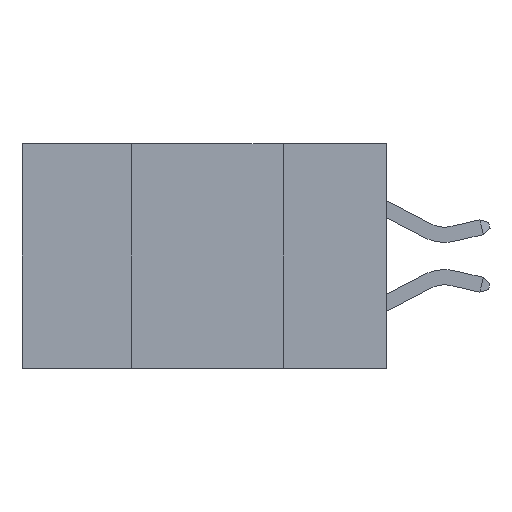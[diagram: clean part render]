
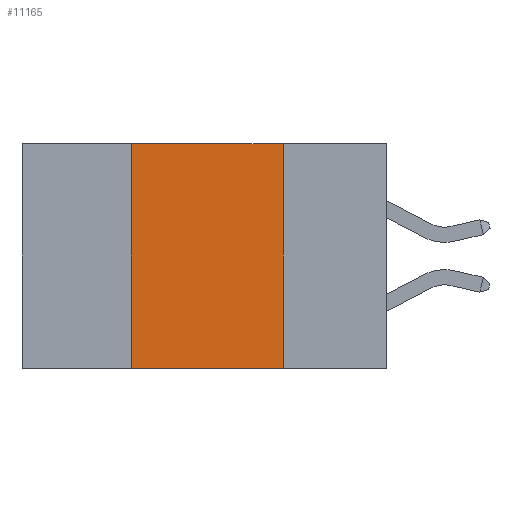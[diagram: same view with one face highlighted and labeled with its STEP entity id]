
A CAD part, left-side view. The second image highlights one B-rep face of the part: STEP entity #11165.
In plain terms, the highlighted planar face has unit normal (-1, 0, 0).
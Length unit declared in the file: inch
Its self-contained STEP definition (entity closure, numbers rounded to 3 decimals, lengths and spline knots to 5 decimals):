
#757 = VERTEX_POINT ( 'NONE', #3958 ) ;
#1578 = CARTESIAN_POINT ( 'NONE',  ( 0., 0.42, 0. ) ) ;
#1702 = LINE ( 'NONE', #13558, #7494 ) ;
#1704 = EDGE_LOOP ( 'NONE', ( #15202, #9391, #8829, #2153 ) ) ;
#2134 = CARTESIAN_POINT ( 'NONE',  ( 0., 0.6, 0. ) ) ;
#2153 = ORIENTED_EDGE ( 'NONE', *, *, #13921, .T. ) ;
#2189 = DIRECTION ( 'NONE',  ( 0., 0., -1. ) ) ;
#2686 = LINE ( 'NONE', #14157, #6401 ) ;
#3408 = DIRECTION ( 'NONE',  ( 1., 0., 0. ) ) ;
#3524 = VECTOR ( 'NONE', #10139, 39.37008 ) ;
#3958 = CARTESIAN_POINT ( 'NONE',  ( 0., 0.17, -0.37 ) ) ;
#5371 = CARTESIAN_POINT ( 'NONE',  ( 0., 0.6, -0.37 ) ) ;
#6296 = AXIS2_PLACEMENT_3D ( 'NONE', #2134, #3408, #11788 ) ;
#6401 = VECTOR ( 'NONE', #7159, 39.37008 ) ;
#6788 = LINE ( 'NONE', #5371, #3524 ) ;
#7139 = EDGE_CURVE ( 'NONE', #10209, #757, #11795, .T. ) ;
#7159 = DIRECTION ( 'NONE',  ( 0., 0., 1. ) ) ;
#7176 = VERTEX_POINT ( 'NONE', #11000 ) ;
#7494 = VECTOR ( 'NONE', #13507, 39.37008 ) ;
#7526 = CARTESIAN_POINT ( 'NONE',  ( 0., 0.17, 0. ) ) ;
#8829 = ORIENTED_EDGE ( 'NONE', *, *, #14829, .F. ) ;
#8831 = EDGE_CURVE ( 'NONE', #9405, #10209, #1702, .T. ) ;
#8929 = CARTESIAN_POINT ( 'NONE',  ( 0., 0.17, 0. ) ) ;
#9391 = ORIENTED_EDGE ( 'NONE', *, *, #8831, .F. ) ;
#9405 = VERTEX_POINT ( 'NONE', #1578 ) ;
#9433 = PLANE ( 'NONE',  #6296 ) ;
#9640 = FACE_OUTER_BOUND ( 'NONE', #1704, .T. ) ;
#10139 = DIRECTION ( 'NONE',  ( 0., -1., 0. ) ) ;
#10209 = VERTEX_POINT ( 'NONE', #7526 ) ;
#11000 = CARTESIAN_POINT ( 'NONE',  ( 0., 0.42, -0.37 ) ) ;
#11165 = ADVANCED_FACE ( 'NONE', ( #9640 ), #9433, .F. ) ;
#11788 = DIRECTION ( 'NONE',  ( 0., 0., -1. ) ) ;
#11795 = LINE ( 'NONE', #8929, #14872 ) ;
#13507 = DIRECTION ( 'NONE',  ( 0., -1., 0. ) ) ;
#13558 = CARTESIAN_POINT ( 'NONE',  ( 0., 0.6, 0. ) ) ;
#13921 = EDGE_CURVE ( 'NONE', #7176, #757, #6788, .T. ) ;
#14157 = CARTESIAN_POINT ( 'NONE',  ( 0., 0.42, 0. ) ) ;
#14829 = EDGE_CURVE ( 'NONE', #7176, #9405, #2686, .T. ) ;
#14872 = VECTOR ( 'NONE', #2189, 39.37008 ) ;
#15202 = ORIENTED_EDGE ( 'NONE', *, *, #7139, .F. ) ;
